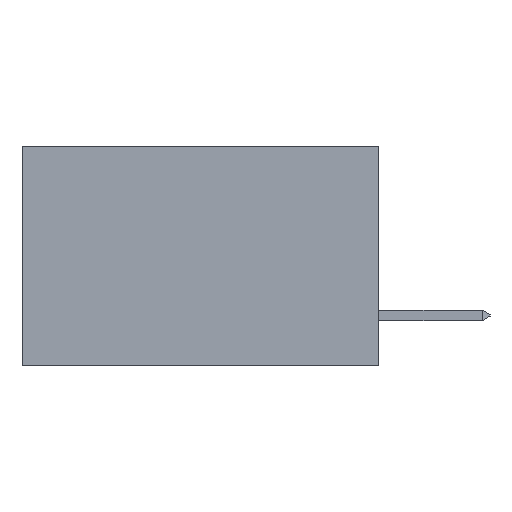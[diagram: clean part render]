
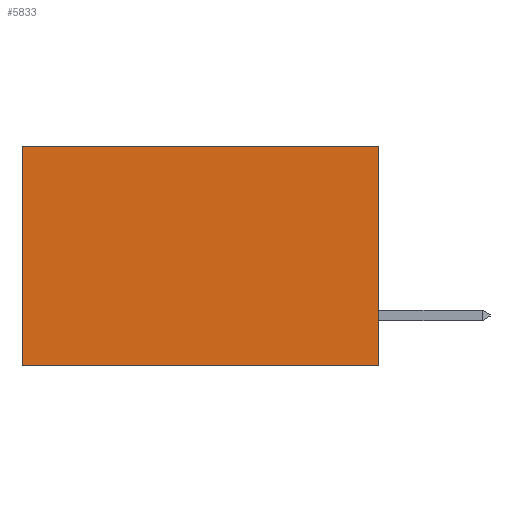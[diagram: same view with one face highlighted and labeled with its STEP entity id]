
A CAD part, left-side view. The second image highlights one B-rep face of the part: STEP entity #5833.
In plain terms, the highlighted planar face has unit normal (-1, 0, 0).
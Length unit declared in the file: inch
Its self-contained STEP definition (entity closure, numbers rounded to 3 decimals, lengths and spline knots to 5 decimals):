
#482 = EDGE_CURVE ( 'NONE', #11889, #13415, #13693, .T. ) ;
#1244 = VECTOR ( 'NONE', #22176, 39.37008 ) ;
#1287 = VERTEX_POINT ( 'NONE', #18527 ) ;
#2707 = LINE ( 'NONE', #14902, #19034 ) ;
#4454 = VECTOR ( 'NONE', #7411, 39.37008 ) ;
#4483 = EDGE_CURVE ( 'NONE', #13415, #19147, #18530, .T. ) ;
#5008 = EDGE_CURVE ( 'NONE', #1287, #19147, #2707, .T. ) ;
#5668 = ORIENTED_EDGE ( 'NONE', *, *, #4483, .F. ) ;
#5833 = ADVANCED_FACE ( 'NONE', ( #8004 ), #21140, .F. ) ;
#7055 = ORIENTED_EDGE ( 'NONE', *, *, #19550, .T. ) ;
#7411 = DIRECTION ( 'NONE',  ( 0., 1., 0. ) ) ;
#7412 = CARTESIAN_POINT ( 'NONE',  ( 0.2615, 0., 0. ) ) ;
#8004 = FACE_OUTER_BOUND ( 'NONE', #21930, .T. ) ;
#9947 = VECTOR ( 'NONE', #13748, 39.37008 ) ;
#10163 = CARTESIAN_POINT ( 'NONE',  ( 0.2615, 0., 0. ) ) ;
#11889 = VERTEX_POINT ( 'NONE', #7412 ) ;
#13415 = VERTEX_POINT ( 'NONE', #22324 ) ;
#13693 = LINE ( 'NONE', #18376, #9947 ) ;
#13748 = DIRECTION ( 'NONE',  ( 0., 0., -1. ) ) ;
#14580 = DIRECTION ( 'NONE',  ( 0., 0., -1. ) ) ;
#14902 = CARTESIAN_POINT ( 'NONE',  ( 0.2615, 0.6, -0.37 ) ) ;
#16229 = AXIS2_PLACEMENT_3D ( 'NONE', #21062, #21039, #21034 ) ;
#17547 = ORIENTED_EDGE ( 'NONE', *, *, #482, .F. ) ;
#18376 = CARTESIAN_POINT ( 'NONE',  ( 0.2615, 0., -0.37 ) ) ;
#18527 = CARTESIAN_POINT ( 'NONE',  ( 0.2615, 0.6, 0. ) ) ;
#18530 = LINE ( 'NONE', #20594, #4454 ) ;
#18974 = LINE ( 'NONE', #10163, #1244 ) ;
#19034 = VECTOR ( 'NONE', #14580, 39.37008 ) ;
#19147 = VERTEX_POINT ( 'NONE', #21077 ) ;
#19550 = EDGE_CURVE ( 'NONE', #11889, #1287, #18974, .T. ) ;
#20594 = CARTESIAN_POINT ( 'NONE',  ( 0.2615, 0., -0.37 ) ) ;
#21034 = DIRECTION ( 'NONE',  ( 0., 0., -1. ) ) ;
#21039 = DIRECTION ( 'NONE',  ( 1., 0., 0. ) ) ;
#21062 = CARTESIAN_POINT ( 'NONE',  ( 0.2615, 0., -0.37 ) ) ;
#21077 = CARTESIAN_POINT ( 'NONE',  ( 0.2615, 0.6, -0.37 ) ) ;
#21140 = PLANE ( 'NONE',  #16229 ) ;
#21930 = EDGE_LOOP ( 'NONE', ( #22170, #5668, #17547, #7055 ) ) ;
#22170 = ORIENTED_EDGE ( 'NONE', *, *, #5008, .T. ) ;
#22176 = DIRECTION ( 'NONE',  ( 0., 1., 0. ) ) ;
#22324 = CARTESIAN_POINT ( 'NONE',  ( 0.2615, 0., -0.37 ) ) ;
